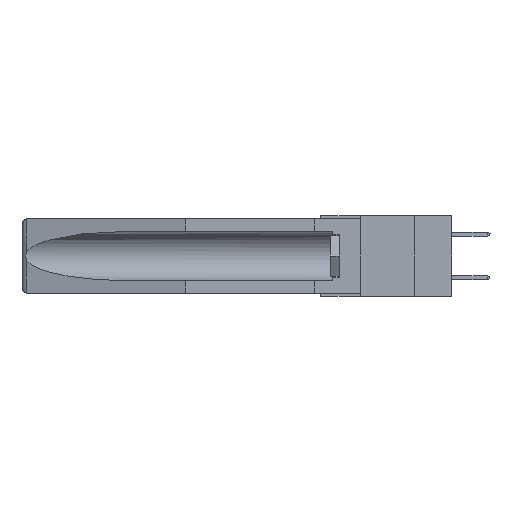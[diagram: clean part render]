
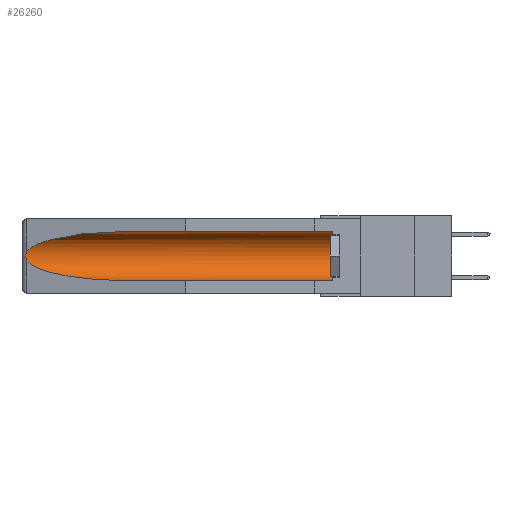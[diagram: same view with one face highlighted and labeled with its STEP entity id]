
A CAD part, left-side view. The second image highlights one B-rep face of the part: STEP entity #26260.
In plain terms, the highlighted cylindrical face has radius 2.857 mm (diameter 5.715 mm), a partial arc.
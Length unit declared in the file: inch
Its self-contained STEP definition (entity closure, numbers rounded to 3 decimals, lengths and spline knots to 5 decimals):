
#12 = CARTESIAN_POINT ( 'NONE',  ( 0.26537, 1.52718, -0.19328 ) ) ;
#66 = CARTESIAN_POINT ( 'NONE',  ( 0.2675, 1.53308, -0.17534 ) ) ;
#271 = CARTESIAN_POINT ( 'NONE',  ( 0.26537, 1.52718, -0.19328 ) ) ;
#979 = VERTEX_POINT ( 'NONE', #19378 ) ;
#2457 = CARTESIAN_POINT ( 'NONE',  ( 0.26597, 1.5296, -0.19026 ) ) ;
#2543 = CARTESIAN_POINT ( 'NONE',  ( 0.155, -0.30754, -0.1715 ) ) ;
#2828 = VERTEX_POINT ( 'NONE', #13913 ) ;
#2928 = DIRECTION ( 'NONE',  ( 0., 1., 0. ) ) ;
#3538 = CARTESIAN_POINT ( 'NONE',  ( 0.26537, 1.52718, -0.14972 ) ) ;
#4205 = DIRECTION ( 'NONE',  ( 0., -1., 0. ) ) ;
#4412 = DIRECTION ( 'NONE',  ( 0., 0., 1. ) ) ;
#4910 = FACE_OUTER_BOUND ( 'NONE', #9220, .T. ) ;
#5132 = EDGE_CURVE ( 'NONE', #979, #2828, #27281, .T. ) ;
#5655 = CARTESIAN_POINT ( 'NONE',  ( 0.155, 1.07973, -0.059 ) ) ;
#5889 = DIRECTION ( 'NONE',  ( 0., 1., 0. ) ) ;
#6989 = EDGE_CURVE ( 'NONE', #7037, #25532, #27505, .T. ) ;
#7037 = VERTEX_POINT ( 'NONE', #29998 ) ;
#7050 = AXIS2_PLACEMENT_3D ( 'NONE', #23510, #4205, #4412 ) ;
#7113 = VECTOR ( 'NONE', #5889, 39.37008 ) ;
#8978 =( BOUNDED_CURVE ( )  B_SPLINE_CURVE ( 3, ( #12, #12261, #9644, #9441 ),
 .UNSPECIFIED., .F., .F. ) 
 B_SPLINE_CURVE_WITH_KNOTS ( ( 4, 4 ),
 ( 0.1948, 1.5708 ),
 .UNSPECIFIED. ) 
 CURVE ( )  GEOMETRIC_REPRESENTATION_ITEM ( )  RATIONAL_B_SPLINE_CURVE ( ( 1., 0.848, 0.848, 1. ) ) 
 REPRESENTATION_ITEM ( '' )  );
#9220 = EDGE_LOOP ( 'NONE', ( #20060, #25501, #15437, #23549, #13188, #17945 ) ) ;
#9441 = CARTESIAN_POINT ( 'NONE',  ( 0.155, 1.07973, -0.284 ) ) ;
#9489 = VERTEX_POINT ( 'NONE', #10694 ) ;
#9644 = CARTESIAN_POINT ( 'NONE',  ( 0.21114, 1.30732, -0.284 ) ) ;
#9817 = CARTESIAN_POINT ( 'NONE',  ( 0.26655, 1.53094, -0.18657 ) ) ;
#10618 = CARTESIAN_POINT ( 'NONE',  ( 0.25451, 1.48313, -0.09465 ) ) ;
#10694 = CARTESIAN_POINT ( 'NONE',  ( 0.26537, 1.52718, -0.19328 ) ) ;
#11252 = VERTEX_POINT ( 'NONE', #14438 ) ;
#11752 = EDGE_CURVE ( 'NONE', #25532, #11252, #11846, .T. ) ;
#11846 =( BOUNDED_CURVE ( )  B_SPLINE_CURVE ( 3, ( #5655, #24822, #10618, #3538 ),
 .UNSPECIFIED., .F., .F. ) 
 B_SPLINE_CURVE_WITH_KNOTS ( ( 4, 4 ),
 ( 4.71239, 6.08839 ),
 .UNSPECIFIED. ) 
 CURVE ( )  GEOMETRIC_REPRESENTATION_ITEM ( )  RATIONAL_B_SPLINE_CURVE ( ( 1., 0.848, 0.848, 1. ) ) 
 REPRESENTATION_ITEM ( '' )  );
#12119 = CARTESIAN_POINT ( 'NONE',  ( 0.2673, 1.5327, -0.16383 ) ) ;
#12261 = CARTESIAN_POINT ( 'NONE',  ( 0.25451, 1.48313, -0.24835 ) ) ;
#13188 = ORIENTED_EDGE ( 'NONE', *, *, #17463, .T. ) ;
#13429 = CARTESIAN_POINT ( 'NONE',  ( 0.155, 1.07973, -0.059 ) ) ;
#13913 = CARTESIAN_POINT ( 'NONE',  ( 0.155, 1.07973, -0.284 ) ) ;
#14293 = CARTESIAN_POINT ( 'NONE',  ( 0.26654, 1.53092, -0.15636 ) ) ;
#14438 = CARTESIAN_POINT ( 'NONE',  ( 0.26537, 1.52718, -0.14972 ) ) ;
#15437 = ORIENTED_EDGE ( 'NONE', *, *, #19116, .T. ) ;
#17163 = AXIS2_PLACEMENT_3D ( 'NONE', #2543, #28652, #28344 ) ;
#17463 = EDGE_CURVE ( 'NONE', #979, #7037, #27540, .T. ) ;
#17714 = CARTESIAN_POINT ( 'NONE',  ( 0.155, -0.30754, -0.059 ) ) ;
#17945 = ORIENTED_EDGE ( 'NONE', *, *, #6989, .T. ) ;
#19116 = EDGE_CURVE ( 'NONE', #9489, #2828, #8978, .T. ) ;
#19378 = CARTESIAN_POINT ( 'NONE',  ( 0.155, 0.126, -0.284 ) ) ;
#20060 = ORIENTED_EDGE ( 'NONE', *, *, #11752, .T. ) ;
#21351 = CARTESIAN_POINT ( 'NONE',  ( 0.2673, 1.53269, -0.17917 ) ) ;
#23099 = CYLINDRICAL_SURFACE ( 'NONE', #17163, 0.1125 ) ;
#23247 = B_SPLINE_CURVE_WITH_KNOTS ( 'NONE', 3,
 ( #24029, #23820, #14293, #12119, #28778, #66, #21351, #9817, #2457, #271 ),
 .UNSPECIFIED., .F., .F.,
 ( 4, 2, 2, 2, 4 ),
 ( 0., 0.00029, 0.00058, 0.00087, 0.00117 ),
 .UNSPECIFIED. ) ;
#23510 = CARTESIAN_POINT ( 'NONE',  ( 0.155, 0.126, -0.1715 ) ) ;
#23549 = ORIENTED_EDGE ( 'NONE', *, *, #5132, .F. ) ;
#23820 = CARTESIAN_POINT ( 'NONE',  ( 0.26597, 1.52961, -0.15275 ) ) ;
#24029 = CARTESIAN_POINT ( 'NONE',  ( 0.26537, 1.52718, -0.14972 ) ) ;
#24822 = CARTESIAN_POINT ( 'NONE',  ( 0.21114, 1.30732, -0.059 ) ) ;
#25501 = ORIENTED_EDGE ( 'NONE', *, *, #30067, .T. ) ;
#25532 = VERTEX_POINT ( 'NONE', #13429 ) ;
#26169 = VECTOR ( 'NONE', #2928, 39.37008 ) ;
#26260 = ADVANCED_FACE ( 'NONE', ( #4910 ), #23099, .F. ) ;
#26471 = CARTESIAN_POINT ( 'NONE',  ( 0.155, -0.30754, -0.284 ) ) ;
#27281 = LINE ( 'NONE', #26471, #26169 ) ;
#27505 = LINE ( 'NONE', #17714, #7113 ) ;
#27540 = CIRCLE ( 'NONE', #7050, 0.1125 ) ;
#28344 = DIRECTION ( 'NONE',  ( 0., 0., 1. ) ) ;
#28652 = DIRECTION ( 'NONE',  ( 0., 1., 0. ) ) ;
#28778 = CARTESIAN_POINT ( 'NONE',  ( 0.2675, 1.53308, -0.16763 ) ) ;
#29998 = CARTESIAN_POINT ( 'NONE',  ( 0.155, 0.126, -0.059 ) ) ;
#30067 = EDGE_CURVE ( 'NONE', #11252, #9489, #23247, .T. ) ;
